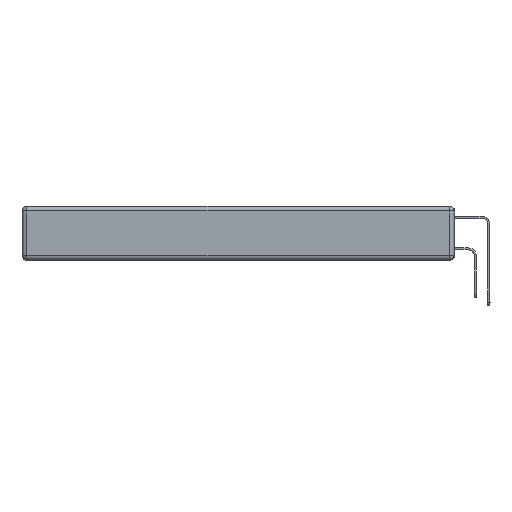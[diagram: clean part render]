
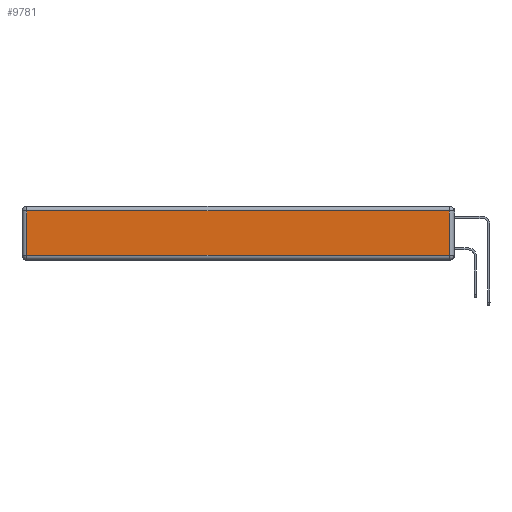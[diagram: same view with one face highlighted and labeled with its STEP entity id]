
A CAD part, left-side view. The second image highlights one B-rep face of the part: STEP entity #9781.
In plain terms, the highlighted planar face has unit normal (-1, 0, 0).
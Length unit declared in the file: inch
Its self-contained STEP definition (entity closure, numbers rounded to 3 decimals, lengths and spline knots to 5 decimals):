
#592 = VERTEX_POINT ( 'NONE', #2191 ) ;
#708 = EDGE_CURVE ( 'NONE', #592, #5160, #16663, .T. ) ;
#1862 = EDGE_CURVE ( 'NONE', #5160, #3366, #19254, .T. ) ;
#1921 = VECTOR ( 'NONE', #4769, 39.37008 ) ;
#2183 = PLANE ( 'NONE',  #17677 ) ;
#2191 = CARTESIAN_POINT ( 'NONE',  ( 0., 2.72, -0.03 ) ) ;
#2220 = ORIENTED_EDGE ( 'NONE', *, *, #19356, .T. ) ;
#2555 = LINE ( 'NONE', #8869, #15619 ) ;
#2693 = DIRECTION ( 'NONE',  ( 0., 0., -1. ) ) ;
#3366 = VERTEX_POINT ( 'NONE', #7533 ) ;
#4769 = DIRECTION ( 'NONE',  ( 0., 0., 1. ) ) ;
#4811 = VECTOR ( 'NONE', #2693, 39.37008 ) ;
#5160 = VERTEX_POINT ( 'NONE', #6381 ) ;
#5405 = ORIENTED_EDGE ( 'NONE', *, *, #19755, .T. ) ;
#5441 = VECTOR ( 'NONE', #14746, 39.37008 ) ;
#6381 = CARTESIAN_POINT ( 'NONE',  ( 0., 2.72, -0.313 ) ) ;
#6558 = DIRECTION ( 'NONE',  ( -1., 0., 0. ) ) ;
#6888 = CARTESIAN_POINT ( 'NONE',  ( 0., 0., -0.313 ) ) ;
#7533 = CARTESIAN_POINT ( 'NONE',  ( 0., 0.03, -0.313 ) ) ;
#8869 = CARTESIAN_POINT ( 'NONE',  ( 0., 2.75, -0.03 ) ) ;
#9167 = DIRECTION ( 'NONE',  ( 0., 1., 0. ) ) ;
#9781 = ADVANCED_FACE ( 'NONE', ( #11227 ), #2183, .T. ) ;
#11127 = CARTESIAN_POINT ( 'NONE',  ( 0., 0., -0.343 ) ) ;
#11227 = FACE_OUTER_BOUND ( 'NONE', #13957, .T. ) ;
#12146 = CARTESIAN_POINT ( 'NONE',  ( 0., 2.72, -0.343 ) ) ;
#12699 = CARTESIAN_POINT ( 'NONE',  ( 0., 0.03, -0.343 ) ) ;
#13347 = VERTEX_POINT ( 'NONE', #17135 ) ;
#13957 = EDGE_LOOP ( 'NONE', ( #19492, #5405, #2220, #17051 ) ) ;
#14746 = DIRECTION ( 'NONE',  ( 0., -1., 0. ) ) ;
#15619 = VECTOR ( 'NONE', #9167, 39.37008 ) ;
#15674 = LINE ( 'NONE', #12699, #1921 ) ;
#16663 = LINE ( 'NONE', #12146, #4811 ) ;
#17051 = ORIENTED_EDGE ( 'NONE', *, *, #708, .T. ) ;
#17135 = CARTESIAN_POINT ( 'NONE',  ( 0., 0.03, -0.03 ) ) ;
#17375 = DIRECTION ( 'NONE',  ( 0., 0., 1. ) ) ;
#17677 = AXIS2_PLACEMENT_3D ( 'NONE', #11127, #6558, #17375 ) ;
#19254 = LINE ( 'NONE', #6888, #5441 ) ;
#19356 = EDGE_CURVE ( 'NONE', #13347, #592, #2555, .T. ) ;
#19492 = ORIENTED_EDGE ( 'NONE', *, *, #1862, .T. ) ;
#19755 = EDGE_CURVE ( 'NONE', #3366, #13347, #15674, .T. ) ;
